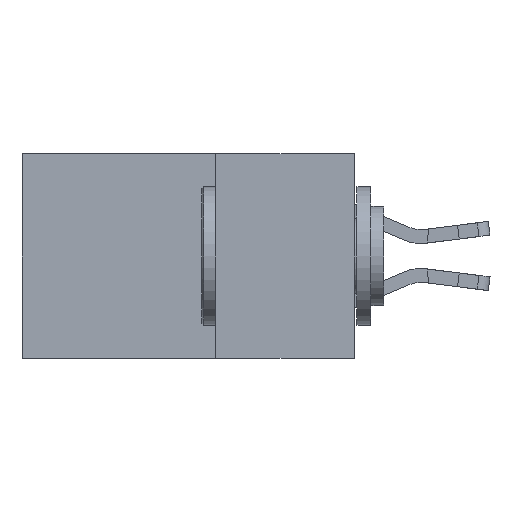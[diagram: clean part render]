
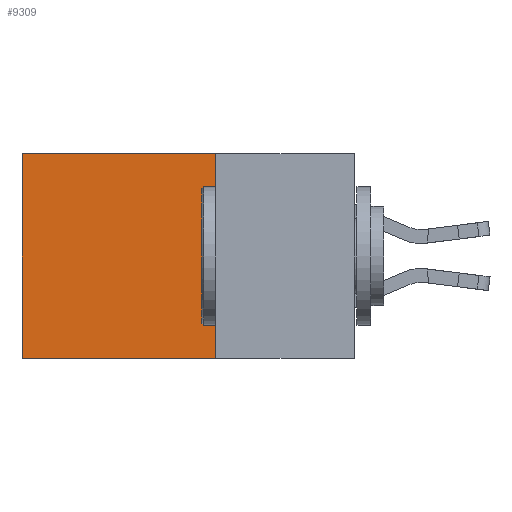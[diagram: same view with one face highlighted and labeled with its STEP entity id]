
A CAD part, left-side view. The second image highlights one B-rep face of the part: STEP entity #9309.
In plain terms, the highlighted planar face has unit normal (-1, 0, 0).
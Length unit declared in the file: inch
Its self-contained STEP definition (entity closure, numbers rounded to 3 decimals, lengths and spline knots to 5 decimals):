
#840 = VERTEX_POINT ( 'NONE', #8477 ) ;
#1294 = DIRECTION ( 'NONE',  ( 0., 0., -1. ) ) ;
#1306 = FACE_OUTER_BOUND ( 'NONE', #2361, .T. ) ;
#1487 = EDGE_CURVE ( 'NONE', #840, #9825, #6040, .T. ) ;
#2187 = LINE ( 'NONE', #3000, #9310 ) ;
#2361 = EDGE_LOOP ( 'NONE', ( #6705, #9070, #3493, #6470 ) ) ;
#3000 = CARTESIAN_POINT ( 'NONE',  ( 0.2615, 0.25, 0. ) ) ;
#3076 = CARTESIAN_POINT ( 'NONE',  ( 0.2615, 0.25, -0.37 ) ) ;
#3493 = ORIENTED_EDGE ( 'NONE', *, *, #1487, .F. ) ;
#3562 = VERTEX_POINT ( 'NONE', #11253 ) ;
#3722 = EDGE_CURVE ( 'NONE', #4627, #3562, #5574, .T. ) ;
#4446 = CARTESIAN_POINT ( 'NONE',  ( 0.2615, 0.25, -0.37 ) ) ;
#4627 = VERTEX_POINT ( 'NONE', #11981 ) ;
#5313 = VECTOR ( 'NONE', #9797, 39.37008 ) ;
#5390 = LINE ( 'NONE', #7519, #12080 ) ;
#5574 = LINE ( 'NONE', #6200, #5313 ) ;
#6040 = LINE ( 'NONE', #11625, #10505 ) ;
#6200 = CARTESIAN_POINT ( 'NONE',  ( 0.2615, 0.6, -0.37 ) ) ;
#6470 = ORIENTED_EDGE ( 'NONE', *, *, #7270, .T. ) ;
#6705 = ORIENTED_EDGE ( 'NONE', *, *, #3722, .T. ) ;
#7086 = DIRECTION ( 'NONE',  ( 1., 0., 0. ) ) ;
#7270 = EDGE_CURVE ( 'NONE', #840, #4627, #2187, .T. ) ;
#7519 = CARTESIAN_POINT ( 'NONE',  ( 0.2615, 0.25, -0.37 ) ) ;
#8428 = DIRECTION ( 'NONE',  ( 0., 1., 0. ) ) ;
#8477 = CARTESIAN_POINT ( 'NONE',  ( 0.2615, 0.25, 0. ) ) ;
#8934 = EDGE_CURVE ( 'NONE', #9825, #3562, #5390, .T. ) ;
#9070 = ORIENTED_EDGE ( 'NONE', *, *, #8934, .F. ) ;
#9309 = ADVANCED_FACE ( 'NONE', ( #1306 ), #11476, .F. ) ;
#9310 = VECTOR ( 'NONE', #9381, 39.37008 ) ;
#9381 = DIRECTION ( 'NONE',  ( 0., 1., 0. ) ) ;
#9797 = DIRECTION ( 'NONE',  ( 0., 0., -1. ) ) ;
#9825 = VERTEX_POINT ( 'NONE', #3076 ) ;
#9921 = DIRECTION ( 'NONE',  ( 0., 0., -1. ) ) ;
#10505 = VECTOR ( 'NONE', #9921, 39.37008 ) ;
#11253 = CARTESIAN_POINT ( 'NONE',  ( 0.2615, 0.6, -0.37 ) ) ;
#11476 = PLANE ( 'NONE',  #11534 ) ;
#11534 = AXIS2_PLACEMENT_3D ( 'NONE', #4446, #7086, #1294 ) ;
#11625 = CARTESIAN_POINT ( 'NONE',  ( 0.2615, 0.25, -0.37 ) ) ;
#11981 = CARTESIAN_POINT ( 'NONE',  ( 0.2615, 0.6, 0. ) ) ;
#12080 = VECTOR ( 'NONE', #8428, 39.37008 ) ;
